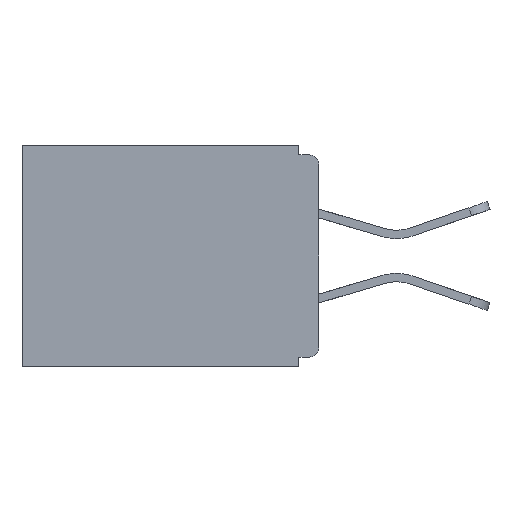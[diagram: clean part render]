
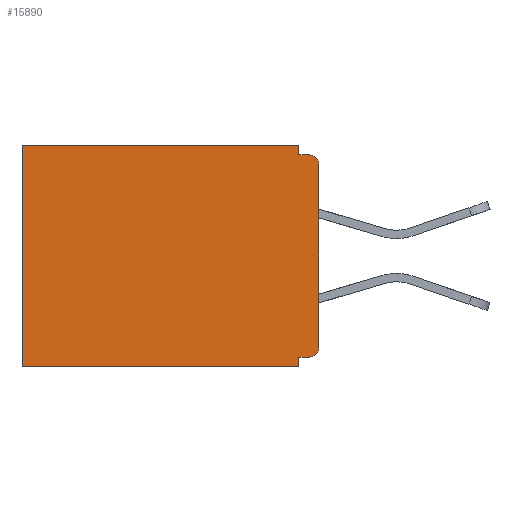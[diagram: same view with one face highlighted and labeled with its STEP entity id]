
A CAD part, left-side view. The second image highlights one B-rep face of the part: STEP entity #15890.
In plain terms, the highlighted planar face has unit normal (-1, 0, 0).
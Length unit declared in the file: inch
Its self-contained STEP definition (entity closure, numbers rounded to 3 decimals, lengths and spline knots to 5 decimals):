
#50 = DIRECTION ( 'NONE',  ( 0., 1., 0. ) ) ;
#402 = CARTESIAN_POINT ( 'NONE',  ( 0.298, 0.031, -0.015 ) ) ;
#685 = AXIS2_PLACEMENT_3D ( 'NONE', #11666, #2567, #16928 ) ;
#830 = CARTESIAN_POINT ( 'NONE',  ( 0.298, 0.031, -0.343 ) ) ;
#1723 = CARTESIAN_POINT ( 'NONE',  ( 0.298, 0., -0.313 ) ) ;
#1751 = CARTESIAN_POINT ( 'NONE',  ( 0.298, 0., -0.03 ) ) ;
#1762 = CARTESIAN_POINT ( 'NONE',  ( 0.298, 0.031, -0.343 ) ) ;
#1995 = ORIENTED_EDGE ( 'NONE', *, *, #10667, .F. ) ;
#2048 = LINE ( 'NONE', #8631, #17994 ) ;
#2375 = CARTESIAN_POINT ( 'NONE',  ( 0.298, 0., 0. ) ) ;
#2567 = DIRECTION ( 'NONE',  ( -1., 0., 0. ) ) ;
#3150 = ORIENTED_EDGE ( 'NONE', *, *, #7519, .T. ) ;
#3211 = ORIENTED_EDGE ( 'NONE', *, *, #16248, .F. ) ;
#3245 = DIRECTION ( 'NONE',  ( 0., 0., -1. ) ) ;
#3281 = EDGE_CURVE ( 'NONE', #19341, #7647, #8616, .T. ) ;
#3432 = VECTOR ( 'NONE', #20708, 39.37008 ) ;
#3695 = VERTEX_POINT ( 'NONE', #4940 ) ;
#3824 = ORIENTED_EDGE ( 'NONE', *, *, #20734, .T. ) ;
#3943 = DIRECTION ( 'NONE',  ( 0., 0., -1. ) ) ;
#4186 = LINE ( 'NONE', #11149, #14745 ) ;
#4291 = CARTESIAN_POINT ( 'NONE',  ( 0.298, 0.031, -0.328 ) ) ;
#4641 = EDGE_LOOP ( 'NONE', ( #8282, #18264, #5319, #14116, #3150, #12045, #3211, #1995, #3824, #14894 ) ) ;
#4779 = CIRCLE ( 'NONE', #16397, 0.015 ) ;
#4940 = CARTESIAN_POINT ( 'NONE',  ( 0.298, 0.46, 0. ) ) ;
#5026 = EDGE_CURVE ( 'NONE', #14562, #17136, #8824, .T. ) ;
#5319 = ORIENTED_EDGE ( 'NONE', *, *, #5026, .F. ) ;
#6778 = CARTESIAN_POINT ( 'NONE',  ( 0.298, 0.015, -0.328 ) ) ;
#6982 = CARTESIAN_POINT ( 'NONE',  ( 0.298, 0.015, -0.313 ) ) ;
#7081 = CARTESIAN_POINT ( 'NONE',  ( 0.298, 0., 0. ) ) ;
#7114 = EDGE_CURVE ( 'NONE', #14562, #3695, #21871, .T. ) ;
#7220 = CARTESIAN_POINT ( 'NONE',  ( 0.298, 0.46, -0.343 ) ) ;
#7519 = EDGE_CURVE ( 'NONE', #3695, #9887, #4186, .T. ) ;
#7647 = VERTEX_POINT ( 'NONE', #1723 ) ;
#8282 = ORIENTED_EDGE ( 'NONE', *, *, #23114, .T. ) ;
#8616 = LINE ( 'NONE', #7081, #10035 ) ;
#8631 = CARTESIAN_POINT ( 'NONE',  ( 0.298, 0., -0.328 ) ) ;
#8824 = LINE ( 'NONE', #830, #3432 ) ;
#9019 = VECTOR ( 'NONE', #9923, 39.37008 ) ;
#9887 = VERTEX_POINT ( 'NONE', #7220 ) ;
#9923 = DIRECTION ( 'NONE',  ( 0., 1., 0. ) ) ;
#10035 = VECTOR ( 'NONE', #20056, 39.37008 ) ;
#10667 = EDGE_CURVE ( 'NONE', #23190, #21121, #2048, .T. ) ;
#11149 = CARTESIAN_POINT ( 'NONE',  ( 0.298, 0.46, 0. ) ) ;
#11294 = AXIS2_PLACEMENT_3D ( 'NONE', #19859, #21947, #21712 ) ;
#11666 = CARTESIAN_POINT ( 'NONE',  ( 0.298, 0.015, -0.03 ) ) ;
#12045 = ORIENTED_EDGE ( 'NONE', *, *, #22529, .F. ) ;
#12540 = DIRECTION ( 'NONE',  ( 0., 1., 0. ) ) ;
#12689 = VECTOR ( 'NONE', #50, 39.37008 ) ;
#12879 = DIRECTION ( 'NONE',  ( 0., 0., -1. ) ) ;
#13836 = CARTESIAN_POINT ( 'NONE',  ( 0.298, 0.031, -0.343 ) ) ;
#14116 = ORIENTED_EDGE ( 'NONE', *, *, #7114, .T. ) ;
#14262 = VECTOR ( 'NONE', #16667, 39.37008 ) ;
#14562 = VERTEX_POINT ( 'NONE', #22094 ) ;
#14707 = CIRCLE ( 'NONE', #685, 0.015 ) ;
#14745 = VECTOR ( 'NONE', #3943, 39.37008 ) ;
#14755 = CARTESIAN_POINT ( 'NONE',  ( 0.298, 0., -0.015 ) ) ;
#14894 = ORIENTED_EDGE ( 'NONE', *, *, #3281, .F. ) ;
#15890 = ADVANCED_FACE ( 'NONE', ( #16471 ), #17617, .F. ) ;
#16248 = EDGE_CURVE ( 'NONE', #21121, #19041, #22162, .T. ) ;
#16397 = AXIS2_PLACEMENT_3D ( 'NONE', #6982, #19551, #3245 ) ;
#16471 = FACE_OUTER_BOUND ( 'NONE', #4641, .T. ) ;
#16667 = DIRECTION ( 'NONE',  ( 0., -1., 0. ) ) ;
#16928 = DIRECTION ( 'NONE',  ( 0., 0., -1. ) ) ;
#17136 = VERTEX_POINT ( 'NONE', #402 ) ;
#17427 = VERTEX_POINT ( 'NONE', #21200 ) ;
#17617 = PLANE ( 'NONE',  #11294 ) ;
#17849 = VECTOR ( 'NONE', #12879, 39.37008 ) ;
#17994 = VECTOR ( 'NONE', #12540, 39.37008 ) ;
#18264 = ORIENTED_EDGE ( 'NONE', *, *, #20306, .F. ) ;
#19041 = VERTEX_POINT ( 'NONE', #13836 ) ;
#19341 = VERTEX_POINT ( 'NONE', #1751 ) ;
#19495 = LINE ( 'NONE', #23560, #12689 ) ;
#19551 = DIRECTION ( 'NONE',  ( -1., 0., 0. ) ) ;
#19859 = CARTESIAN_POINT ( 'NONE',  ( 0.298, 0., 0. ) ) ;
#20056 = DIRECTION ( 'NONE',  ( 0., 0., -1. ) ) ;
#20306 = EDGE_CURVE ( 'NONE', #17136, #17427, #23391, .T. ) ;
#20708 = DIRECTION ( 'NONE',  ( 0., 0., -1. ) ) ;
#20734 = EDGE_CURVE ( 'NONE', #23190, #7647, #4779, .T. ) ;
#21121 = VERTEX_POINT ( 'NONE', #4291 ) ;
#21200 = CARTESIAN_POINT ( 'NONE',  ( 0.298, 0.015, -0.015 ) ) ;
#21712 = DIRECTION ( 'NONE',  ( 0., 0., -1. ) ) ;
#21871 = LINE ( 'NONE', #2375, #9019 ) ;
#21947 = DIRECTION ( 'NONE',  ( 1., 0., 0. ) ) ;
#22094 = CARTESIAN_POINT ( 'NONE',  ( 0.298, 0.031, 0. ) ) ;
#22162 = LINE ( 'NONE', #1762, #17849 ) ;
#22529 = EDGE_CURVE ( 'NONE', #19041, #9887, #19495, .T. ) ;
#23114 = EDGE_CURVE ( 'NONE', #19341, #17427, #14707, .T. ) ;
#23190 = VERTEX_POINT ( 'NONE', #6778 ) ;
#23391 = LINE ( 'NONE', #14755, #14262 ) ;
#23560 = CARTESIAN_POINT ( 'NONE',  ( 0.298, 0., -0.343 ) ) ;
